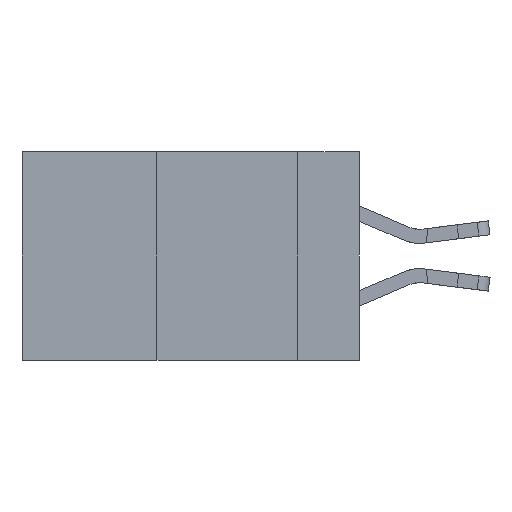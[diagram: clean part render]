
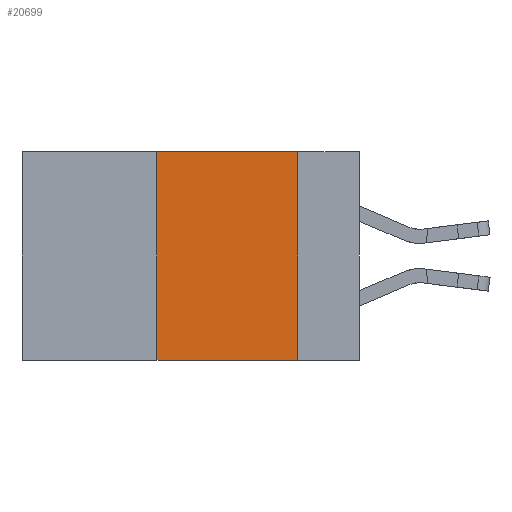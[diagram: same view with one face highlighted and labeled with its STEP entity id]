
A CAD part, left-side view. The second image highlights one B-rep face of the part: STEP entity #20699.
In plain terms, the highlighted planar face has unit normal (-1, 0, 0).
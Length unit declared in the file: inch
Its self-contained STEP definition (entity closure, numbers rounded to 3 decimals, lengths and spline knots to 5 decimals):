
#589 = DIRECTION ( 'NONE',  ( 0., 0., -1. ) ) ;
#1304 = ORIENTED_EDGE ( 'NONE', *, *, #20737, .T. ) ;
#3426 = VECTOR ( 'NONE', #5601, 39.37008 ) ;
#3811 = CARTESIAN_POINT ( 'NONE',  ( 0., 0.36, 0. ) ) ;
#4200 = CARTESIAN_POINT ( 'NONE',  ( 0., 0.11, 0. ) ) ;
#4270 = CARTESIAN_POINT ( 'NONE',  ( 0., 0.36, 0. ) ) ;
#5601 = DIRECTION ( 'NONE',  ( 0., -1., 0. ) ) ;
#6128 = ORIENTED_EDGE ( 'NONE', *, *, #6552, .F. ) ;
#6552 = EDGE_CURVE ( 'NONE', #9582, #21883, #17538, .T. ) ;
#8284 = VECTOR ( 'NONE', #17965, 39.37008 ) ;
#9294 = LINE ( 'NONE', #14911, #18140 ) ;
#9333 = CARTESIAN_POINT ( 'NONE',  ( 0., 0.6, 0. ) ) ;
#9426 = EDGE_CURVE ( 'NONE', #21614, #9582, #13558, .T. ) ;
#9493 = PLANE ( 'NONE',  #16934 ) ;
#9582 = VERTEX_POINT ( 'NONE', #4270 ) ;
#10364 = DIRECTION ( 'NONE',  ( 0., 0., -1. ) ) ;
#10395 = FACE_OUTER_BOUND ( 'NONE', #19746, .T. ) ;
#11273 = DIRECTION ( 'NONE',  ( 1., 0., 0. ) ) ;
#11594 = VERTEX_POINT ( 'NONE', #14675 ) ;
#13558 = LINE ( 'NONE', #3811, #8284 ) ;
#14675 = CARTESIAN_POINT ( 'NONE',  ( 0., 0.11, -0.37 ) ) ;
#14911 = CARTESIAN_POINT ( 'NONE',  ( 0., 0.6, -0.37 ) ) ;
#15332 = ORIENTED_EDGE ( 'NONE', *, *, #22754, .F. ) ;
#15880 = CARTESIAN_POINT ( 'NONE',  ( 0., 0.36, -0.37 ) ) ;
#16934 = AXIS2_PLACEMENT_3D ( 'NONE', #21881, #11273, #589 ) ;
#17538 = LINE ( 'NONE', #9333, #3426 ) ;
#17965 = DIRECTION ( 'NONE',  ( 0., 0., 1. ) ) ;
#18140 = VECTOR ( 'NONE', #18474, 39.37008 ) ;
#18150 = VECTOR ( 'NONE', #10364, 39.37008 ) ;
#18474 = DIRECTION ( 'NONE',  ( 0., -1., 0. ) ) ;
#18740 = LINE ( 'NONE', #22683, #18150 ) ;
#18811 = ORIENTED_EDGE ( 'NONE', *, *, #9426, .F. ) ;
#19746 = EDGE_LOOP ( 'NONE', ( #15332, #6128, #18811, #1304 ) ) ;
#20699 = ADVANCED_FACE ( 'NONE', ( #10395 ), #9493, .F. ) ;
#20737 = EDGE_CURVE ( 'NONE', #21614, #11594, #9294, .T. ) ;
#21614 = VERTEX_POINT ( 'NONE', #15880 ) ;
#21881 = CARTESIAN_POINT ( 'NONE',  ( 0., 0.6, 0. ) ) ;
#21883 = VERTEX_POINT ( 'NONE', #4200 ) ;
#22683 = CARTESIAN_POINT ( 'NONE',  ( 0., 0.11, 0. ) ) ;
#22754 = EDGE_CURVE ( 'NONE', #21883, #11594, #18740, .T. ) ;
